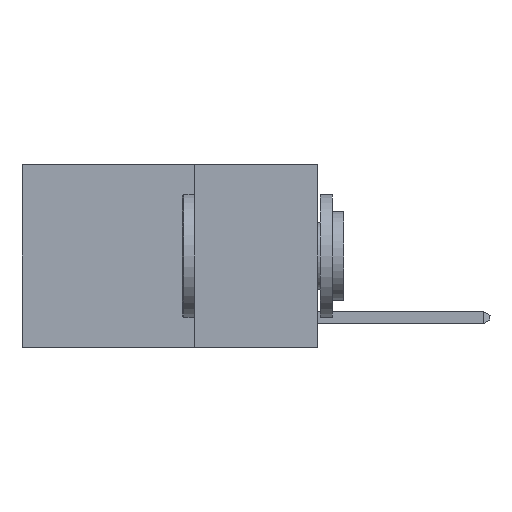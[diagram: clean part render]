
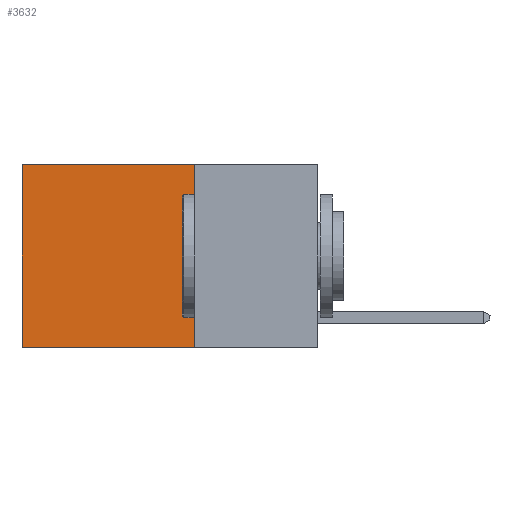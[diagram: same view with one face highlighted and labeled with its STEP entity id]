
A CAD part, left-side view. The second image highlights one B-rep face of the part: STEP entity #3632.
In plain terms, the highlighted planar face has unit normal (-1, 0, 0).
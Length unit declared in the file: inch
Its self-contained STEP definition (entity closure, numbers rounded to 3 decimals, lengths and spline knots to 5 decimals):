
#547 = CARTESIAN_POINT ( 'NONE',  ( 0.2625, 0.25, 0. ) ) ;
#680 = CARTESIAN_POINT ( 'NONE',  ( 0.2625, 0.25, -0.37 ) ) ;
#781 = VECTOR ( 'NONE', #5076, 39.37008 ) ;
#940 = VERTEX_POINT ( 'NONE', #7387 ) ;
#1306 = DIRECTION ( 'NONE',  ( 0., 0., -1. ) ) ;
#1713 = AXIS2_PLACEMENT_3D ( 'NONE', #3648, #6688, #5874 ) ;
#1754 = DIRECTION ( 'NONE',  ( 0., 0., -1. ) ) ;
#2051 = VERTEX_POINT ( 'NONE', #4886 ) ;
#2173 = FACE_OUTER_BOUND ( 'NONE', #5992, .T. ) ;
#2263 = EDGE_CURVE ( 'NONE', #4154, #8994, #8198, .T. ) ;
#2272 = PLANE ( 'NONE',  #1713 ) ;
#3132 = ORIENTED_EDGE ( 'NONE', *, *, #2263, .F. ) ;
#3581 = CARTESIAN_POINT ( 'NONE',  ( 0.2625, 0.6, -0.37 ) ) ;
#3632 = ADVANCED_FACE ( 'NONE', ( #2173 ), #2272, .F. ) ;
#3648 = CARTESIAN_POINT ( 'NONE',  ( 0.2625, 0.25, 0. ) ) ;
#3842 = DIRECTION ( 'NONE',  ( 0., 1., 0. ) ) ;
#4154 = VERTEX_POINT ( 'NONE', #7462 ) ;
#4885 = EDGE_CURVE ( 'NONE', #2051, #940, #8852, .T. ) ;
#4886 = CARTESIAN_POINT ( 'NONE',  ( 0.2625, 0.25, 0. ) ) ;
#5076 = DIRECTION ( 'NONE',  ( 0., 1., 0. ) ) ;
#5118 = EDGE_CURVE ( 'NONE', #2051, #4154, #7795, .T. ) ;
#5468 = VECTOR ( 'NONE', #1306, 39.37008 ) ;
#5874 = DIRECTION ( 'NONE',  ( 0., 0., -1. ) ) ;
#5992 = EDGE_LOOP ( 'NONE', ( #7715, #3132, #6647, #7908 ) ) ;
#6142 = CARTESIAN_POINT ( 'NONE',  ( 0.2625, 0.25, 0. ) ) ;
#6406 = LINE ( 'NONE', #7989, #5468 ) ;
#6647 = ORIENTED_EDGE ( 'NONE', *, *, #5118, .F. ) ;
#6688 = DIRECTION ( 'NONE',  ( 1., 0., 0. ) ) ;
#7344 = EDGE_CURVE ( 'NONE', #940, #8994, #6406, .T. ) ;
#7387 = CARTESIAN_POINT ( 'NONE',  ( 0.2625, 0.6, 0. ) ) ;
#7462 = CARTESIAN_POINT ( 'NONE',  ( 0.2625, 0.25, -0.37 ) ) ;
#7715 = ORIENTED_EDGE ( 'NONE', *, *, #7344, .T. ) ;
#7795 = LINE ( 'NONE', #6142, #8259 ) ;
#7908 = ORIENTED_EDGE ( 'NONE', *, *, #4885, .T. ) ;
#7989 = CARTESIAN_POINT ( 'NONE',  ( 0.2625, 0.6, 0. ) ) ;
#8198 = LINE ( 'NONE', #680, #9655 ) ;
#8259 = VECTOR ( 'NONE', #1754, 39.37008 ) ;
#8852 = LINE ( 'NONE', #547, #781 ) ;
#8994 = VERTEX_POINT ( 'NONE', #3581 ) ;
#9655 = VECTOR ( 'NONE', #3842, 39.37008 ) ;
